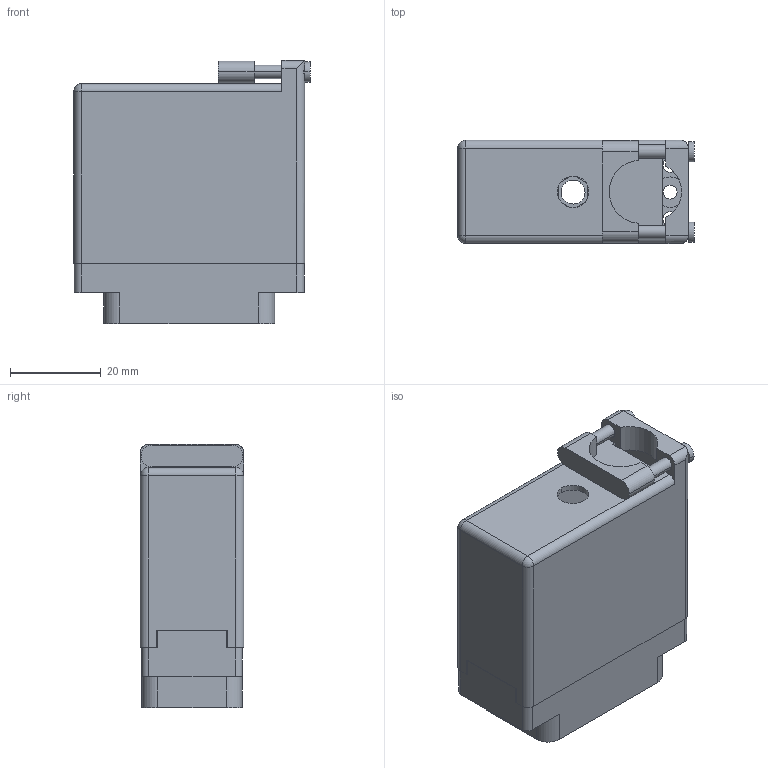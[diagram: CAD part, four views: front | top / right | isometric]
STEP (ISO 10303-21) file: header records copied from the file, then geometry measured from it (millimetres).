
FILE_DESCRIPTION (( 'STEP AP203' ), '1' );
FILE_NAME ('516-038-500-560.STEP', '2020-03-09T20:43:59', ( '' ), ( '' ), 'SwSTEP 2.0', 'SolidWorks 2016', '' );
FILE_SCHEMA (( 'CONFIG_CONTROL_DESIGN' ));
Length unit declared in the file: inch
Products named in the file (4): 516-292-001_500 Contact; 516-038-500-560; 516-230-001_Metal - 038 Top Entry; 516 Plug Insulator_038
Assembly tree (40 placements, depth 2):
  516-038-500-560
    516 Plug Insulator_038
    516-292-001_500 Contact  x38
    516-230-001_Metal - 038 Top Entry
Bounding box: 52.27 x 22.83 x 58.12 mm (x, y, z)
Volume: 19090.5 mm3; surface area: 32450 mm2
Topology: 40 solids, 40 shells, 3837 faces, 11136 edges, 7392 vertices
Faces by surface type: plane 2308, cylinder 1297, bspline 228, cone 2, sphere 2
Entity records: 35957 total; most frequent: CARTESIAN_POINT 6379, ORIENTED_EDGE 5988, DIRECTION 5818, EDGE_CURVE 2994, VECTOR 2214, LINE 2214, VERTEX_POINT 1990, AXIS2_PLACEMENT_3D 1802
